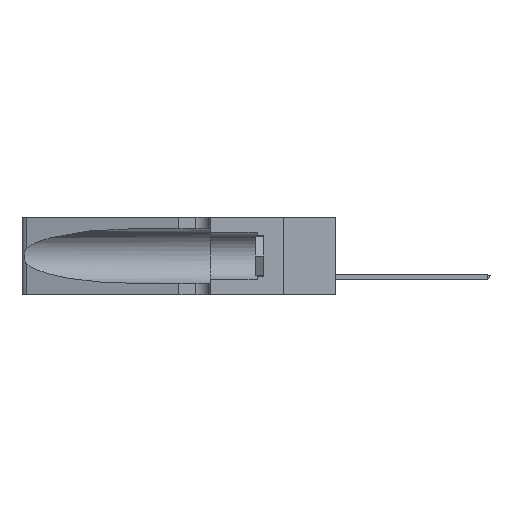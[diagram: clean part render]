
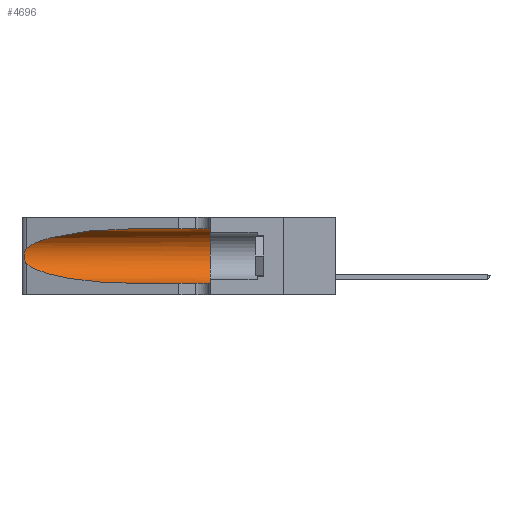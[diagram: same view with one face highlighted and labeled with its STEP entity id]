
A CAD part, left-side view. The second image highlights one B-rep face of the part: STEP entity #4696.
In plain terms, the highlighted cylindrical face has radius 3.308 mm (diameter 6.617 mm), a partial arc.
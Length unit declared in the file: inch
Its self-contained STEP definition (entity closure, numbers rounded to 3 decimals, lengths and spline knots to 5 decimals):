
#30 =( BOUNDED_CURVE ( )  B_SPLINE_CURVE ( 3, ( #29174, #21303, #10808, #5201 ),
 .UNSPECIFIED., .F., .T. ) 
 B_SPLINE_CURVE_WITH_KNOTS ( ( 4, 4 ),
 ( 3.44316, 4.71239 ),
 .UNSPECIFIED. ) 
 CURVE ( )  GEOMETRIC_REPRESENTATION_ITEM ( )  RATIONAL_B_SPLINE_CURVE ( ( 1., 0.87, 0.87, 1. ) ) 
 REPRESENTATION_ITEM ( '' )  );
#262 = AXIS2_PLACEMENT_3D ( 'NONE', #30088, #772, #19422 ) ;
#304 = EDGE_CURVE ( 'NONE', #10917, #4021, #30, .T. ) ;
#772 = DIRECTION ( 'NONE',  ( 0., 1., 0. ) ) ;
#1927 = DIRECTION ( 'NONE',  ( 0., -1., 0. ) ) ;
#2743 = CARTESIAN_POINT ( 'NONE',  ( 0.1305, 1.61858, 0.31525 ) ) ;
#3699 = CARTESIAN_POINT ( 'NONE',  ( 0.1305, 0.35, 0.31525 ) ) ;
#3794 = ORIENTED_EDGE ( 'NONE', *, *, #16415, .F. ) ;
#4021 = VERTEX_POINT ( 'NONE', #19954 ) ;
#4235 = CARTESIAN_POINT ( 'NONE',  ( 0.1305, 1.61858, 0.05475 ) ) ;
#4696 = ADVANCED_FACE ( 'NONE', ( #29104 ), #25381, .F. ) ;
#5181 = VERTEX_POINT ( 'NONE', #3699 ) ;
#5201 = CARTESIAN_POINT ( 'NONE',  ( 0.1305, 0.72297, 0.05475 ) ) ;
#5866 = ORIENTED_EDGE ( 'NONE', *, *, #13308, .T. ) ;
#6153 = CARTESIAN_POINT ( 'NONE',  ( 0.25639, 1.23184, 0.21858 ) ) ;
#6703 = EDGE_CURVE ( 'NONE', #5181, #28224, #28644, .T. ) ;
#7541 = LINE ( 'NONE', #2743, #19937 ) ;
#8815 = CARTESIAN_POINT ( 'NONE',  ( 0.25555, 1.22994, 0.2215 ) ) ;
#9388 = CARTESIAN_POINT ( 'NONE',  ( 0.26017, 1.23833, 0.17102 ) ) ;
#9854 = LINE ( 'NONE', #4235, #22226 ) ;
#10808 = CARTESIAN_POINT ( 'NONE',  ( 0.18966, 0.96281, 0.05475 ) ) ;
#10917 = VERTEX_POINT ( 'NONE', #31634 ) ;
#12599 = ORIENTED_EDGE ( 'NONE', *, *, #18525, .T. ) ;
#13308 = EDGE_CURVE ( 'NONE', #26295, #29227, #19444, .T. ) ;
#14086 = CARTESIAN_POINT ( 'NONE',  ( 0.25787, 1.23484, 0.2124 ) ) ;
#16293 = CARTESIAN_POINT ( 'NONE',  ( 0.1305, 0.72297, 0.31525 ) ) ;
#16415 = EDGE_CURVE ( 'NONE', #26295, #5181, #7541, .T. ) ;
#16858 = CARTESIAN_POINT ( 'NONE',  ( 0.26075, 1.23896, 0.19203 ) ) ;
#17589 = CARTESIAN_POINT ( 'NONE',  ( 0.1305, 0.72297, 0.31525 ) ) ;
#18525 = EDGE_CURVE ( 'NONE', #29227, #10917, #21984, .T. ) ;
#18733 = ORIENTED_EDGE ( 'NONE', *, *, #304, .T. ) ;
#19054 = CARTESIAN_POINT ( 'NONE',  ( 0.26075, 1.23896, 0.178 ) ) ;
#19422 = DIRECTION ( 'NONE',  ( 0., 0., 1. ) ) ;
#19444 =( BOUNDED_CURVE ( )  B_SPLINE_CURVE ( 3, ( #16293, #19623, #27117, #27490 ),
 .UNSPECIFIED., .F., .T. ) 
 B_SPLINE_CURVE_WITH_KNOTS ( ( 4, 4 ),
 ( 1.5708, 2.84003 ),
 .UNSPECIFIED. ) 
 CURVE ( )  GEOMETRIC_REPRESENTATION_ITEM ( )  RATIONAL_B_SPLINE_CURVE ( ( 1., 0.87, 0.87, 1. ) ) 
 REPRESENTATION_ITEM ( '' )  );
#19623 = CARTESIAN_POINT ( 'NONE',  ( 0.18966, 0.96281, 0.31525 ) ) ;
#19937 = VECTOR ( 'NONE', #26362, 39.37008 ) ;
#19954 = CARTESIAN_POINT ( 'NONE',  ( 0.1305, 0.72297, 0.05475 ) ) ;
#20001 = CARTESIAN_POINT ( 'NONE',  ( 0.25789, 1.23486, 0.15765 ) ) ;
#20396 = CARTESIAN_POINT ( 'NONE',  ( 0.25487, 1.22718, 0.22369 ) ) ;
#21303 = CARTESIAN_POINT ( 'NONE',  ( 0.2373, 1.15595, 0.08982 ) ) ;
#21552 = EDGE_LOOP ( 'NONE', ( #5866, #12599, #18733, #25579, #22178, #3794 ) ) ;
#21984 = B_SPLINE_CURVE_WITH_KNOTS ( 'NONE', 3,
 ( #22062, #8815, #6153, #14086, #32617, #26911, #16858, #19054, #9388, #30202, #20001, #22423, #32864, #27964 ),
 .UNSPECIFIED., .F., .F.,
 ( 4, 2, 2, 2, 2, 2, 4 ),
 ( 0., 0.00027, 0.00053, 0.00107, 0.0016, 0.00187, 0.00214 ),
 .UNSPECIFIED. ) ;
#22062 = CARTESIAN_POINT ( 'NONE',  ( 0.25487, 1.22718, 0.22369 ) ) ;
#22178 = ORIENTED_EDGE ( 'NONE', *, *, #6703, .F. ) ;
#22226 = VECTOR ( 'NONE', #1927, 39.37008 ) ;
#22423 = CARTESIAN_POINT ( 'NONE',  ( 0.25639, 1.23186, 0.15144 ) ) ;
#23252 = AXIS2_PLACEMENT_3D ( 'NONE', #23545, #25848, #30020 ) ;
#23545 = CARTESIAN_POINT ( 'NONE',  ( 0.1305, 1.61858, 0.185 ) ) ;
#25184 = EDGE_CURVE ( 'NONE', #4021, #28224, #9854, .T. ) ;
#25381 = CYLINDRICAL_SURFACE ( 'NONE', #23252, 0.13025 ) ;
#25579 = ORIENTED_EDGE ( 'NONE', *, *, #25184, .T. ) ;
#25848 = DIRECTION ( 'NONE',  ( 0., -1., 0. ) ) ;
#26295 = VERTEX_POINT ( 'NONE', #17589 ) ;
#26362 = DIRECTION ( 'NONE',  ( 0., -1., 0. ) ) ;
#26911 = CARTESIAN_POINT ( 'NONE',  ( 0.26018, 1.23835, 0.19895 ) ) ;
#27117 = CARTESIAN_POINT ( 'NONE',  ( 0.2373, 1.15595, 0.28018 ) ) ;
#27490 = CARTESIAN_POINT ( 'NONE',  ( 0.25487, 1.22718, 0.22369 ) ) ;
#27964 = CARTESIAN_POINT ( 'NONE',  ( 0.25487, 1.22718, 0.14631 ) ) ;
#28224 = VERTEX_POINT ( 'NONE', #32772 ) ;
#28644 = CIRCLE ( 'NONE', #262, 0.13025 ) ;
#29104 = FACE_OUTER_BOUND ( 'NONE', #21552, .T. ) ;
#29174 = CARTESIAN_POINT ( 'NONE',  ( 0.25487, 1.22718, 0.14631 ) ) ;
#29227 = VERTEX_POINT ( 'NONE', #20396 ) ;
#30020 = DIRECTION ( 'NONE',  ( 0., 0., -1. ) ) ;
#30088 = CARTESIAN_POINT ( 'NONE',  ( 0.1305, 0.35, 0.185 ) ) ;
#30202 = CARTESIAN_POINT ( 'NONE',  ( 0.25856, 1.23593, 0.16098 ) ) ;
#31634 = CARTESIAN_POINT ( 'NONE',  ( 0.25487, 1.22718, 0.14631 ) ) ;
#32617 = CARTESIAN_POINT ( 'NONE',  ( 0.25854, 1.2359, 0.20912 ) ) ;
#32772 = CARTESIAN_POINT ( 'NONE',  ( 0.1305, 0.35, 0.05475 ) ) ;
#32864 = CARTESIAN_POINT ( 'NONE',  ( 0.25555, 1.22993, 0.14849 ) ) ;
